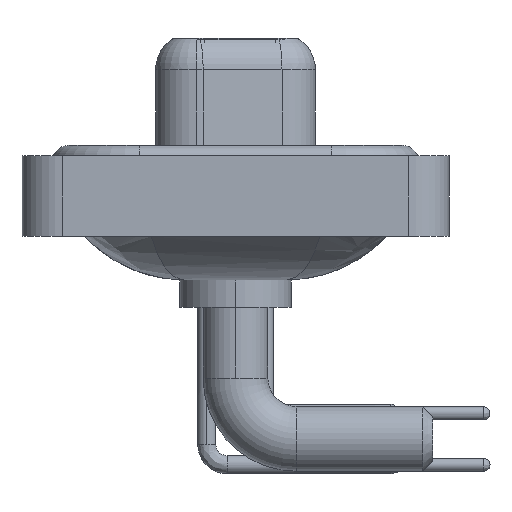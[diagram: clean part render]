
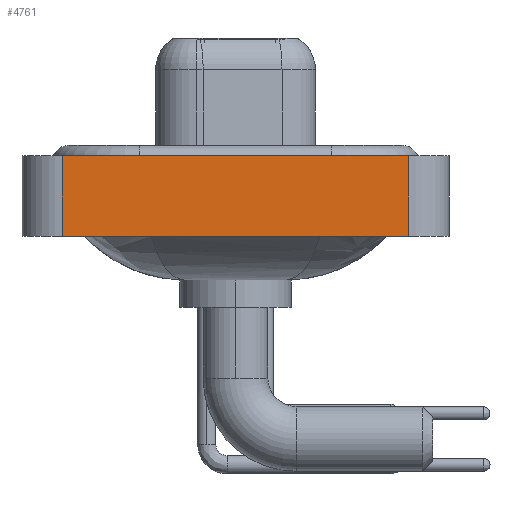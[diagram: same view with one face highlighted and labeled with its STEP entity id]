
A CAD part, left-side view. The second image highlights one B-rep face of the part: STEP entity #4761.
In plain terms, the highlighted planar face has unit normal (-1, 0, 0).
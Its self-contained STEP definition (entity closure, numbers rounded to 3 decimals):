
#327 = VECTOR ( 'NONE', #7571, 1000. ) ;
#874 = DIRECTION ( 'NONE',  ( 0., 0., 1. ) ) ;
#2715 = VERTEX_POINT ( 'NONE', #21700 ) ;
#2724 = CARTESIAN_POINT ( 'NONE',  ( -7.35, -8.55, 0.4 ) ) ;
#2867 = VERTEX_POINT ( 'NONE', #19063 ) ;
#3031 = CARTESIAN_POINT ( 'NONE',  ( -7.35, -8.55, -3.6 ) ) ;
#3147 = EDGE_CURVE ( 'NONE', #2715, #15282, #5803, .T. ) ;
#3448 = AXIS2_PLACEMENT_3D ( 'NONE', #14984, #13259, #6492 ) ;
#3747 = CARTESIAN_POINT ( 'NONE',  ( -7.35, 8.55, -3.6 ) ) ;
#3757 = LINE ( 'NONE', #3031, #13796 ) ;
#4207 = ORIENTED_EDGE ( 'NONE', *, *, #13044, .F. ) ;
#4349 = VERTEX_POINT ( 'NONE', #3747 ) ;
#4761 = ADVANCED_FACE ( 'NONE', ( #13392 ), #17083, .T. ) ;
#5803 = LINE ( 'NONE', #14879, #20320 ) ;
#5968 = CARTESIAN_POINT ( 'NONE',  ( -7.35, -8.55, 0.4 ) ) ;
#6492 = DIRECTION ( 'NONE',  ( 0., 0., 1. ) ) ;
#6902 = ORIENTED_EDGE ( 'NONE', *, *, #17983, .T. ) ;
#7348 = LINE ( 'NONE', #9062, #13399 ) ;
#7571 = DIRECTION ( 'NONE',  ( 0., -1., 0. ) ) ;
#9062 = CARTESIAN_POINT ( 'NONE',  ( -7.35, 8.55, -3.6 ) ) ;
#9875 = EDGE_LOOP ( 'NONE', ( #15474, #4207, #14415, #6902 ) ) ;
#12488 = LINE ( 'NONE', #5968, #327 ) ;
#13044 = EDGE_CURVE ( 'NONE', #2867, #15282, #12488, .T. ) ;
#13259 = DIRECTION ( 'NONE',  ( -1., 0., 0. ) ) ;
#13392 = FACE_OUTER_BOUND ( 'NONE', #9875, .T. ) ;
#13399 = VECTOR ( 'NONE', #19549, 1000. ) ;
#13796 = VECTOR ( 'NONE', #17054, 1000. ) ;
#14415 = ORIENTED_EDGE ( 'NONE', *, *, #16128, .F. ) ;
#14879 = CARTESIAN_POINT ( 'NONE',  ( -7.35, -8.55, -3.6 ) ) ;
#14984 = CARTESIAN_POINT ( 'NONE',  ( -7.35, -8.55, -3.6 ) ) ;
#15282 = VERTEX_POINT ( 'NONE', #2724 ) ;
#15474 = ORIENTED_EDGE ( 'NONE', *, *, #3147, .T. ) ;
#16128 = EDGE_CURVE ( 'NONE', #4349, #2867, #7348, .T. ) ;
#17054 = DIRECTION ( 'NONE',  ( 0., -1., 0. ) ) ;
#17083 = PLANE ( 'NONE',  #3448 ) ;
#17983 = EDGE_CURVE ( 'NONE', #4349, #2715, #3757, .T. ) ;
#19063 = CARTESIAN_POINT ( 'NONE',  ( -7.35, 8.55, 0.4 ) ) ;
#19549 = DIRECTION ( 'NONE',  ( 0., 0., 1. ) ) ;
#20320 = VECTOR ( 'NONE', #874, 1000. ) ;
#21700 = CARTESIAN_POINT ( 'NONE',  ( -7.35, -8.55, -3.6 ) ) ;
